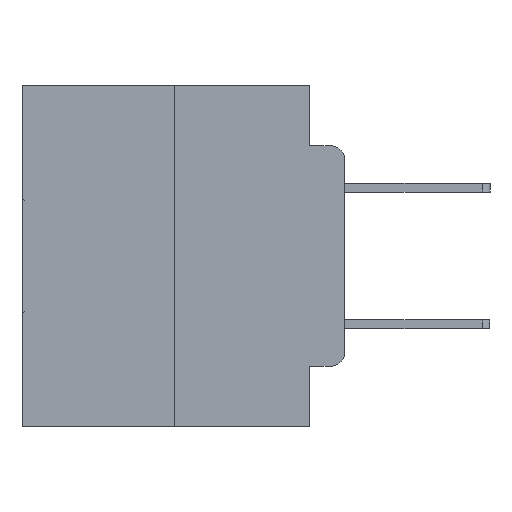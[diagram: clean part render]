
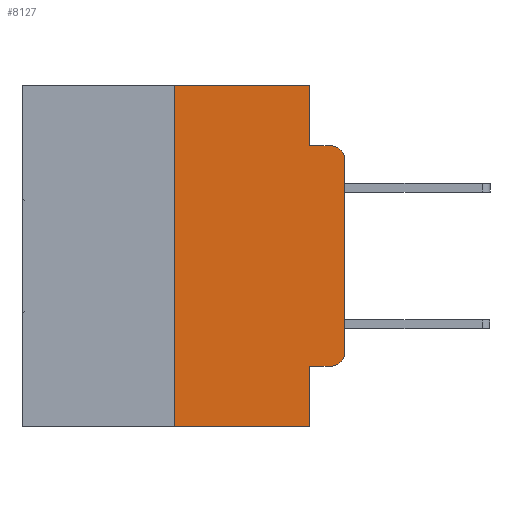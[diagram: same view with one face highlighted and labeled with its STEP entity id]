
A CAD part, left-side view. The second image highlights one B-rep face of the part: STEP entity #8127.
In plain terms, the highlighted planar face has unit normal (-1, 0, 0).
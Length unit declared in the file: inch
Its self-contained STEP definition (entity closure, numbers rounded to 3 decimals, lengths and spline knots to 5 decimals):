
#232 = VERTEX_POINT ( 'NONE', #18273 ) ;
#311 = LINE ( 'NONE', #1273, #23898 ) ;
#320 = EDGE_LOOP ( 'NONE', ( #7936, #21944, #10158, #19329, #14595, #20849, #18409, #29434, #23607, #24703 ) ) ;
#521 = VERTEX_POINT ( 'NONE', #10457 ) ;
#766 = VECTOR ( 'NONE', #24850, 39.37008 ) ;
#917 = EDGE_CURVE ( 'NONE', #521, #23915, #7737, .T. ) ;
#1273 = CARTESIAN_POINT ( 'NONE',  ( 0., 0.473, 0. ) ) ;
#1782 = VERTEX_POINT ( 'NONE', #24812 ) ;
#2056 = VECTOR ( 'NONE', #7742, 39.37008 ) ;
#2294 = VERTEX_POINT ( 'NONE', #18907 ) ;
#2345 = DIRECTION ( 'NONE',  ( 0., 0., -1. ) ) ;
#2381 = VECTOR ( 'NONE', #14059, 39.37008 ) ;
#2484 = LINE ( 'NONE', #21765, #23456 ) ;
#3061 = CARTESIAN_POINT ( 'NONE',  ( 0., 0.02, -0.1085 ) ) ;
#3105 = LINE ( 'NONE', #25892, #2381 ) ;
#3287 = VECTOR ( 'NONE', #6791, 39.37008 ) ;
#4194 = CARTESIAN_POINT ( 'NONE',  ( 0., 0., -0.1085 ) ) ;
#4455 = CIRCLE ( 'NONE', #29050, 0.02 ) ;
#5426 = DIRECTION ( 'NONE',  ( 0., 0., -1. ) ) ;
#6092 = DIRECTION ( 'NONE',  ( 0., 0., 1. ) ) ;
#6688 = CARTESIAN_POINT ( 'NONE',  ( 0., 0.051, -0.0885 ) ) ;
#6791 = DIRECTION ( 'NONE',  ( 0., -1., 0. ) ) ;
#7657 = DIRECTION ( 'NONE',  ( 0., -1., 0. ) ) ;
#7737 = LINE ( 'NONE', #10739, #766 ) ;
#7742 = DIRECTION ( 'NONE',  ( 0., 0., -1. ) ) ;
#7778 = EDGE_CURVE ( 'NONE', #25787, #18144, #20798, .T. ) ;
#7936 = ORIENTED_EDGE ( 'NONE', *, *, #917, .T. ) ;
#8127 = ADVANCED_FACE ( 'NONE', ( #22993 ), #20691, .F. ) ;
#8249 = DIRECTION ( 'NONE',  ( -1., 0., 0. ) ) ;
#8306 = VERTEX_POINT ( 'NONE', #28405 ) ;
#8697 = AXIS2_PLACEMENT_3D ( 'NONE', #23075, #27824, #13746 ) ;
#8911 = VECTOR ( 'NONE', #6092, 39.37008 ) ;
#9530 = LINE ( 'NONE', #6688, #3287 ) ;
#9822 = VERTEX_POINT ( 'NONE', #19747 ) ;
#10158 = ORIENTED_EDGE ( 'NONE', *, *, #18783, .F. ) ;
#10457 = CARTESIAN_POINT ( 'NONE',  ( 0., 0., -0.3915 ) ) ;
#10739 = CARTESIAN_POINT ( 'NONE',  ( 0., 0., 0. ) ) ;
#10765 = AXIS2_PLACEMENT_3D ( 'NONE', #3061, #19454, #5426 ) ;
#11452 = EDGE_CURVE ( 'NONE', #9822, #18144, #3105, .T. ) ;
#12556 = EDGE_CURVE ( 'NONE', #9822, #24505, #15140, .T. ) ;
#12578 = CARTESIAN_POINT ( 'NONE',  ( 0., 0.25, 0. ) ) ;
#12904 = CARTESIAN_POINT ( 'NONE',  ( 0., 0.051, -0.5 ) ) ;
#13746 = DIRECTION ( 'NONE',  ( 0., 0., -1. ) ) ;
#14059 = DIRECTION ( 'NONE',  ( 0., -1., 0. ) ) ;
#14425 = CIRCLE ( 'NONE', #10765, 0.02 ) ;
#14595 = ORIENTED_EDGE ( 'NONE', *, *, #29178, .F. ) ;
#15140 = LINE ( 'NONE', #12578, #8911 ) ;
#15332 = DIRECTION ( 'NONE',  ( 0., -1., 0. ) ) ;
#17208 = EDGE_CURVE ( 'NONE', #2294, #1782, #28059, .T. ) ;
#18144 = VERTEX_POINT ( 'NONE', #12904 ) ;
#18273 = CARTESIAN_POINT ( 'NONE',  ( 0., 0.02, -0.4115 ) ) ;
#18409 = ORIENTED_EDGE ( 'NONE', *, *, #11452, .T. ) ;
#18726 = CARTESIAN_POINT ( 'NONE',  ( 0., 0.051, 0. ) ) ;
#18783 = EDGE_CURVE ( 'NONE', #1782, #8306, #9530, .T. ) ;
#18907 = CARTESIAN_POINT ( 'NONE',  ( 0., 0.051, 0. ) ) ;
#19329 = ORIENTED_EDGE ( 'NONE', *, *, #17208, .F. ) ;
#19454 = DIRECTION ( 'NONE',  ( -1., 0., 0. ) ) ;
#19747 = CARTESIAN_POINT ( 'NONE',  ( 0., 0.25, -0.5 ) ) ;
#20691 = PLANE ( 'NONE',  #8697 ) ;
#20798 = LINE ( 'NONE', #24229, #2056 ) ;
#20849 = ORIENTED_EDGE ( 'NONE', *, *, #12556, .F. ) ;
#21045 = VECTOR ( 'NONE', #2345, 39.37008 ) ;
#21765 = CARTESIAN_POINT ( 'NONE',  ( 0., 0.051, -0.4115 ) ) ;
#21944 = ORIENTED_EDGE ( 'NONE', *, *, #23578, .T. ) ;
#22993 = FACE_OUTER_BOUND ( 'NONE', #320, .T. ) ;
#23075 = CARTESIAN_POINT ( 'NONE',  ( 0., 0.473, 0. ) ) ;
#23456 = VECTOR ( 'NONE', #7657, 39.37008 ) ;
#23575 = CARTESIAN_POINT ( 'NONE',  ( 0., 0.25, 0. ) ) ;
#23578 = EDGE_CURVE ( 'NONE', #23915, #8306, #14425, .T. ) ;
#23607 = ORIENTED_EDGE ( 'NONE', *, *, #30370, .T. ) ;
#23898 = VECTOR ( 'NONE', #15332, 39.37008 ) ;
#23915 = VERTEX_POINT ( 'NONE', #4194 ) ;
#24162 = EDGE_CURVE ( 'NONE', #232, #521, #4455, .T. ) ;
#24229 = CARTESIAN_POINT ( 'NONE',  ( 0., 0.051, 0. ) ) ;
#24505 = VERTEX_POINT ( 'NONE', #23575 ) ;
#24703 = ORIENTED_EDGE ( 'NONE', *, *, #24162, .T. ) ;
#24720 = DIRECTION ( 'NONE',  ( 0., 0., -1. ) ) ;
#24812 = CARTESIAN_POINT ( 'NONE',  ( 0., 0.051, -0.0885 ) ) ;
#24850 = DIRECTION ( 'NONE',  ( 0., 0., 1. ) ) ;
#25098 = CARTESIAN_POINT ( 'NONE',  ( 0., 0.02, -0.3915 ) ) ;
#25787 = VERTEX_POINT ( 'NONE', #25886 ) ;
#25886 = CARTESIAN_POINT ( 'NONE',  ( 0., 0.051, -0.4115 ) ) ;
#25892 = CARTESIAN_POINT ( 'NONE',  ( 0., 0.473, -0.5 ) ) ;
#27824 = DIRECTION ( 'NONE',  ( 1., 0., 0. ) ) ;
#28059 = LINE ( 'NONE', #18726, #21045 ) ;
#28405 = CARTESIAN_POINT ( 'NONE',  ( 0., 0.02, -0.0885 ) ) ;
#29050 = AXIS2_PLACEMENT_3D ( 'NONE', #25098, #8249, #24720 ) ;
#29178 = EDGE_CURVE ( 'NONE', #24505, #2294, #311, .T. ) ;
#29434 = ORIENTED_EDGE ( 'NONE', *, *, #7778, .F. ) ;
#30370 = EDGE_CURVE ( 'NONE', #25787, #232, #2484, .T. ) ;
